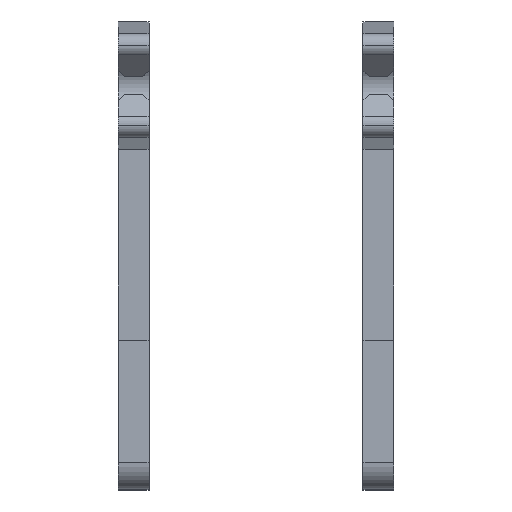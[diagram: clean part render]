
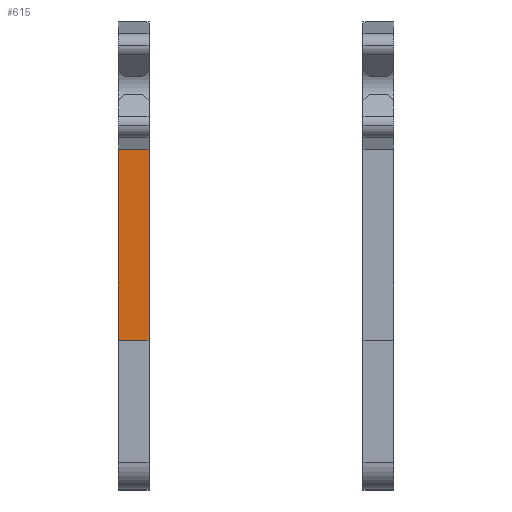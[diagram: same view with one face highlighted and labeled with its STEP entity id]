
A CAD part, top view. The second image highlights one B-rep face of the part: STEP entity #615.
In plain terms, the highlighted planar face has unit normal (0, 0, 1).
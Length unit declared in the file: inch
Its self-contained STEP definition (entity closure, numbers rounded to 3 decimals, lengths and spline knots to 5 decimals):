
#10 = CARTESIAN_POINT ( 'NONE',  ( 0.0125, -0.208, -0.07 ) ) ;
#12 = EDGE_CURVE ( 'NONE', #805, #267, #574, .T. ) ;
#14 = VECTOR ( 'NONE', #1139, 39.37008 ) ;
#112 = ORIENTED_EDGE ( 'NONE', *, *, #696, .F. ) ;
#198 = VECTOR ( 'NONE', #1315, 39.37008 ) ;
#199 = VECTOR ( 'NONE', #560, 39.37008 ) ;
#203 = VERTEX_POINT ( 'NONE', #875 ) ;
#219 = DIRECTION ( 'NONE',  ( 0., 0., -1. ) ) ;
#251 = ORIENTED_EDGE ( 'NONE', *, *, #12, .T. ) ;
#259 = EDGE_CURVE ( 'NONE', #1140, #805, #1224, .T. ) ;
#267 = VERTEX_POINT ( 'NONE', #314 ) ;
#314 = CARTESIAN_POINT ( 'NONE',  ( -0.0125, -0.208, -0.07 ) ) ;
#330 = DIRECTION ( 'NONE',  ( -1., 0., 0. ) ) ;
#367 = LINE ( 'NONE', #1176, #199 ) ;
#387 = CARTESIAN_POINT ( 'NONE',  ( -0.0125, -0.208, -0.07 ) ) ;
#429 = DIRECTION ( 'NONE',  ( -1., 0., 0. ) ) ;
#464 = CARTESIAN_POINT ( 'NONE',  ( 0.0125, -0.208, -0.07 ) ) ;
#476 = EDGE_CURVE ( 'NONE', #1140, #203, #367, .T. ) ;
#521 = FACE_OUTER_BOUND ( 'NONE', #1326, .T. ) ;
#534 = CARTESIAN_POINT ( 'NONE',  ( 0.0125, -0.052, -0.07 ) ) ;
#560 = DIRECTION ( 'NONE',  ( 0., -1., 0. ) ) ;
#574 = LINE ( 'NONE', #387, #14 ) ;
#615 = ADVANCED_FACE ( 'NONE', ( #521 ), #868, .F. ) ;
#674 = CARTESIAN_POINT ( 'NONE',  ( 0.0125, -0.052, -0.07 ) ) ;
#696 = EDGE_CURVE ( 'NONE', #203, #267, #1276, .T. ) ;
#760 = AXIS2_PLACEMENT_3D ( 'NONE', #10, #219, #330 ) ;
#805 = VERTEX_POINT ( 'NONE', #1255 ) ;
#868 = PLANE ( 'NONE',  #760 ) ;
#875 = CARTESIAN_POINT ( 'NONE',  ( 0.0125, -0.208, -0.07 ) ) ;
#1139 = DIRECTION ( 'NONE',  ( 0., -1., 0. ) ) ;
#1140 = VERTEX_POINT ( 'NONE', #534 ) ;
#1176 = CARTESIAN_POINT ( 'NONE',  ( 0.0125, -0.208, -0.07 ) ) ;
#1194 = VECTOR ( 'NONE', #429, 39.37008 ) ;
#1224 = LINE ( 'NONE', #674, #1194 ) ;
#1255 = CARTESIAN_POINT ( 'NONE',  ( -0.0125, -0.052, -0.07 ) ) ;
#1276 = LINE ( 'NONE', #464, #198 ) ;
#1283 = ORIENTED_EDGE ( 'NONE', *, *, #259, .T. ) ;
#1315 = DIRECTION ( 'NONE',  ( -1., 0., 0. ) ) ;
#1326 = EDGE_LOOP ( 'NONE', ( #251, #112, #1337, #1283 ) ) ;
#1337 = ORIENTED_EDGE ( 'NONE', *, *, #476, .F. ) ;
